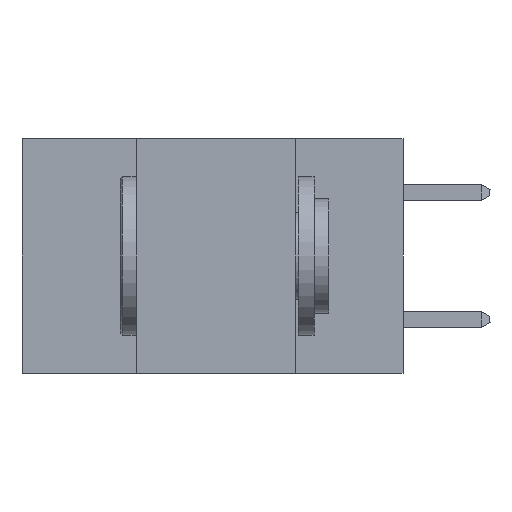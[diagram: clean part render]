
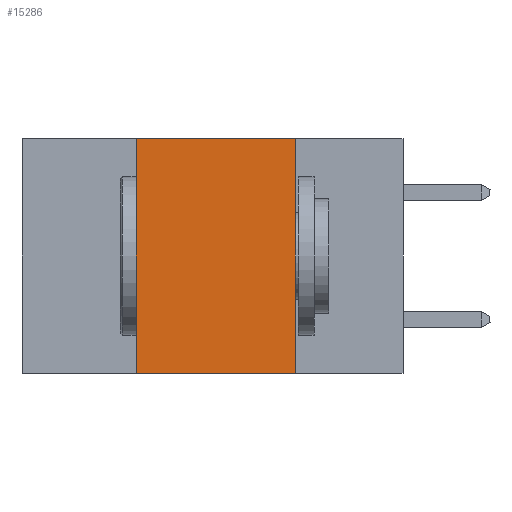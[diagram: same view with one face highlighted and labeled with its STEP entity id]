
A CAD part, left-side view. The second image highlights one B-rep face of the part: STEP entity #15286.
In plain terms, the highlighted planar face has unit normal (-1, 0, 0).
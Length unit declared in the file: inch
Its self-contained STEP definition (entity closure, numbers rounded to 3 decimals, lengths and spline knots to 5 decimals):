
#3502 = DIRECTION ( 'NONE',  ( 0., -1., 0. ) ) ;
#5476 = VECTOR ( 'NONE', #3502, 39.37008 ) ;
#6167 = CARTESIAN_POINT ( 'NONE',  ( 0., 0.42, 0. ) ) ;
#6596 = VERTEX_POINT ( 'NONE', #32125 ) ;
#11642 = EDGE_CURVE ( 'NONE', #14020, #6596, #38482, .T. ) ;
#14020 = VERTEX_POINT ( 'NONE', #6167 ) ;
#14651 = VECTOR ( 'NONE', #32214, 39.37008 ) ;
#15075 = EDGE_CURVE ( 'NONE', #6596, #24037, #18684, .T. ) ;
#15286 = ADVANCED_FACE ( 'NONE', ( #29475 ), #21110, .F. ) ;
#16237 = EDGE_LOOP ( 'NONE', ( #16804, #41003, #32749, #34131 ) ) ;
#16804 = ORIENTED_EDGE ( 'NONE', *, *, #15075, .F. ) ;
#17198 = AXIS2_PLACEMENT_3D ( 'NONE', #17640, #42137, #24887 ) ;
#17634 = EDGE_CURVE ( 'NONE', #34414, #24037, #29252, .T. ) ;
#17640 = CARTESIAN_POINT ( 'NONE',  ( 0., 0.6, 0. ) ) ;
#18684 = LINE ( 'NONE', #26895, #37051 ) ;
#20208 = DIRECTION ( 'NONE',  ( 0., 0., -1. ) ) ;
#21110 = PLANE ( 'NONE',  #17198 ) ;
#22758 = CARTESIAN_POINT ( 'NONE',  ( 0., 0.17, -0.37 ) ) ;
#22760 = LINE ( 'NONE', #27809, #42236 ) ;
#24037 = VERTEX_POINT ( 'NONE', #22758 ) ;
#24887 = DIRECTION ( 'NONE',  ( 0., 0., -1. ) ) ;
#26505 = EDGE_CURVE ( 'NONE', #34414, #14020, #22760, .T. ) ;
#26895 = CARTESIAN_POINT ( 'NONE',  ( 0., 0.17, 0. ) ) ;
#27809 = CARTESIAN_POINT ( 'NONE',  ( 0., 0.42, 0. ) ) ;
#29252 = LINE ( 'NONE', #42062, #14651 ) ;
#29475 = FACE_OUTER_BOUND ( 'NONE', #16237, .T. ) ;
#32125 = CARTESIAN_POINT ( 'NONE',  ( 0., 0.17, 0. ) ) ;
#32214 = DIRECTION ( 'NONE',  ( 0., -1., 0. ) ) ;
#32749 = ORIENTED_EDGE ( 'NONE', *, *, #26505, .F. ) ;
#34100 = CARTESIAN_POINT ( 'NONE',  ( 0., 0.42, -0.37 ) ) ;
#34131 = ORIENTED_EDGE ( 'NONE', *, *, #17634, .T. ) ;
#34414 = VERTEX_POINT ( 'NONE', #34100 ) ;
#37051 = VECTOR ( 'NONE', #20208, 39.37008 ) ;
#38482 = LINE ( 'NONE', #41505, #5476 ) ;
#38830 = DIRECTION ( 'NONE',  ( 0., 0., 1. ) ) ;
#41003 = ORIENTED_EDGE ( 'NONE', *, *, #11642, .F. ) ;
#41505 = CARTESIAN_POINT ( 'NONE',  ( 0., 0.6, 0. ) ) ;
#42062 = CARTESIAN_POINT ( 'NONE',  ( 0., 0.6, -0.37 ) ) ;
#42137 = DIRECTION ( 'NONE',  ( 1., 0., 0. ) ) ;
#42236 = VECTOR ( 'NONE', #38830, 39.37008 ) ;
